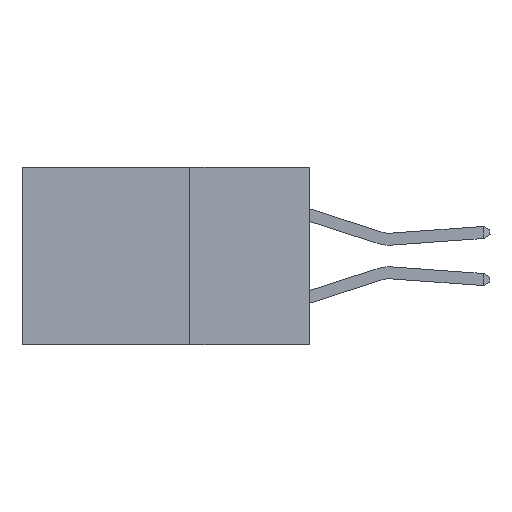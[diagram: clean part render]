
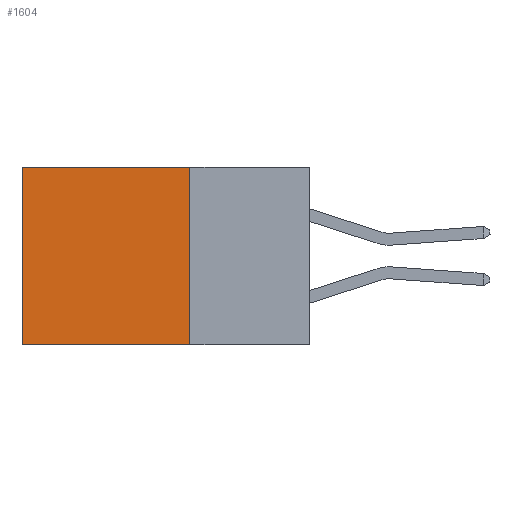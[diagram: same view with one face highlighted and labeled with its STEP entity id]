
A CAD part, left-side view. The second image highlights one B-rep face of the part: STEP entity #1604.
In plain terms, the highlighted planar face has unit normal (-1, 0, 0).
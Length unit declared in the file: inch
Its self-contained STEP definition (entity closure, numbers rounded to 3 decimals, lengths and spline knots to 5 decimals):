
#27 = EDGE_CURVE ( 'NONE', #14055, #2785, #14783, .T. ) ;
#1157 = VECTOR ( 'NONE', #10368, 39.37008 ) ;
#1290 = AXIS2_PLACEMENT_3D ( 'NONE', #10462, #12778, #9293 ) ;
#1604 = ADVANCED_FACE ( 'NONE', ( #4538 ), #3386, .F. ) ;
#2455 = LINE ( 'NONE', #4850, #11836 ) ;
#2785 = VERTEX_POINT ( 'NONE', #13397 ) ;
#2799 = CARTESIAN_POINT ( 'NONE',  ( 0.2615, 0.25, -0.37 ) ) ;
#3032 = ORIENTED_EDGE ( 'NONE', *, *, #14419, .F. ) ;
#3386 = PLANE ( 'NONE',  #1290 ) ;
#3565 = ORIENTED_EDGE ( 'NONE', *, *, #27, .T. ) ;
#3942 = DIRECTION ( 'NONE',  ( 0., 0., -1. ) ) ;
#4538 = FACE_OUTER_BOUND ( 'NONE', #12804, .T. ) ;
#4711 = ORIENTED_EDGE ( 'NONE', *, *, #15057, .T. ) ;
#4850 = CARTESIAN_POINT ( 'NONE',  ( 0.2615, 0.25, 0. ) ) ;
#5522 = LINE ( 'NONE', #5685, #1157 ) ;
#5685 = CARTESIAN_POINT ( 'NONE',  ( 0.2615, 0.25, -0.37 ) ) ;
#5877 = VERTEX_POINT ( 'NONE', #12427 ) ;
#6636 = DIRECTION ( 'NONE',  ( 0., 0., -1. ) ) ;
#7089 = VECTOR ( 'NONE', #3942, 39.37008 ) ;
#7842 = VECTOR ( 'NONE', #6636, 39.37008 ) ;
#8577 = CARTESIAN_POINT ( 'NONE',  ( 0.2615, 0.6, 0. ) ) ;
#9293 = DIRECTION ( 'NONE',  ( 0., 0., -1. ) ) ;
#9459 = EDGE_CURVE ( 'NONE', #5877, #13195, #13330, .T. ) ;
#10368 = DIRECTION ( 'NONE',  ( 0., 1., 0. ) ) ;
#10462 = CARTESIAN_POINT ( 'NONE',  ( 0.2615, 0.25, -0.37 ) ) ;
#10990 = ORIENTED_EDGE ( 'NONE', *, *, #9459, .F. ) ;
#11836 = VECTOR ( 'NONE', #14851, 39.37008 ) ;
#12427 = CARTESIAN_POINT ( 'NONE',  ( 0.2615, 0.25, 0. ) ) ;
#12778 = DIRECTION ( 'NONE',  ( 1., 0., 0. ) ) ;
#12804 = EDGE_LOOP ( 'NONE', ( #3565, #3032, #10990, #4711 ) ) ;
#13195 = VERTEX_POINT ( 'NONE', #2799 ) ;
#13330 = LINE ( 'NONE', #13560, #7089 ) ;
#13397 = CARTESIAN_POINT ( 'NONE',  ( 0.2615, 0.6, -0.37 ) ) ;
#13560 = CARTESIAN_POINT ( 'NONE',  ( 0.2615, 0.25, -0.37 ) ) ;
#13855 = CARTESIAN_POINT ( 'NONE',  ( 0.2615, 0.6, -0.37 ) ) ;
#14055 = VERTEX_POINT ( 'NONE', #8577 ) ;
#14419 = EDGE_CURVE ( 'NONE', #13195, #2785, #5522, .T. ) ;
#14783 = LINE ( 'NONE', #13855, #7842 ) ;
#14851 = DIRECTION ( 'NONE',  ( 0., 1., 0. ) ) ;
#15057 = EDGE_CURVE ( 'NONE', #5877, #14055, #2455, .T. ) ;
